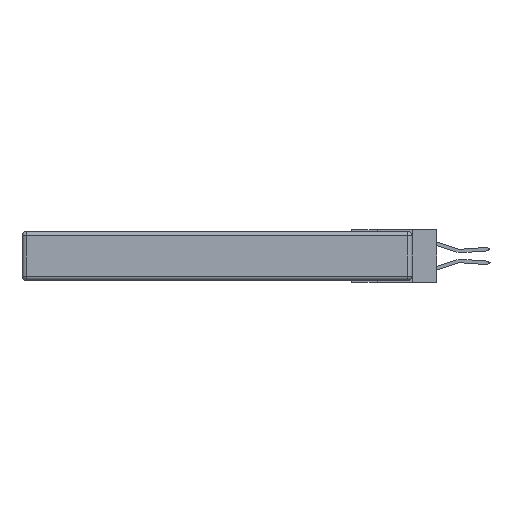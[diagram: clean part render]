
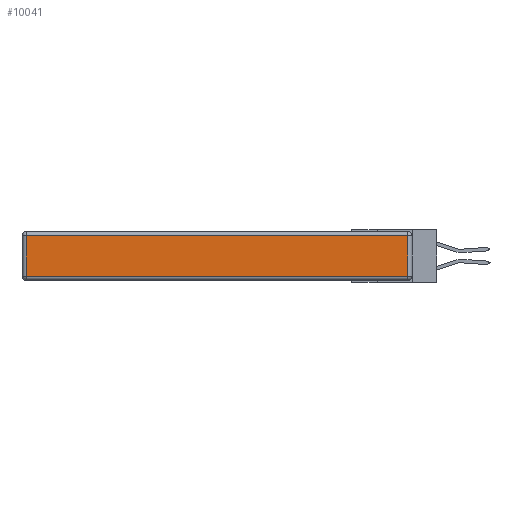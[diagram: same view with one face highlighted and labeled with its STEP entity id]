
A CAD part, left-side view. The second image highlights one B-rep face of the part: STEP entity #10041.
In plain terms, the highlighted planar face has unit normal (-1, 0, 0).
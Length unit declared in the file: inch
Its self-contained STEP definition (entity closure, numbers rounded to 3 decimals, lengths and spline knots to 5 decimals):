
#207 = CARTESIAN_POINT ( 'NONE',  ( 0., 0., -0.343 ) ) ;
#346 = LINE ( 'NONE', #9034, #8412 ) ;
#557 = ORIENTED_EDGE ( 'NONE', *, *, #4192, .T. ) ;
#729 = CARTESIAN_POINT ( 'NONE',  ( 0., 2.75, -0.03 ) ) ;
#798 = VERTEX_POINT ( 'NONE', #8414 ) ;
#1135 = FACE_OUTER_BOUND ( 'NONE', #7737, .T. ) ;
#1770 = DIRECTION ( 'NONE',  ( 0., 1., 0. ) ) ;
#1778 = EDGE_CURVE ( 'NONE', #9830, #3579, #13136, .T. ) ;
#2706 = DIRECTION ( 'NONE',  ( 0., 0., 1. ) ) ;
#3579 = VERTEX_POINT ( 'NONE', #10986 ) ;
#3909 = CARTESIAN_POINT ( 'NONE',  ( 0., 2.72, -0.343 ) ) ;
#4192 = EDGE_CURVE ( 'NONE', #798, #13851, #4459, .T. ) ;
#4459 = LINE ( 'NONE', #3909, #13299 ) ;
#5035 = EDGE_CURVE ( 'NONE', #13851, #9830, #346, .T. ) ;
#5189 = VECTOR ( 'NONE', #2706, 39.37008 ) ;
#6120 = CARTESIAN_POINT ( 'NONE',  ( 0., 0.03, -0.343 ) ) ;
#6155 = ORIENTED_EDGE ( 'NONE', *, *, #5035, .T. ) ;
#6741 = AXIS2_PLACEMENT_3D ( 'NONE', #207, #6930, #10423 ) ;
#6930 = DIRECTION ( 'NONE',  ( -1., 0., 0. ) ) ;
#7737 = EDGE_LOOP ( 'NONE', ( #6155, #11279, #12709, #557 ) ) ;
#8412 = VECTOR ( 'NONE', #10199, 39.37008 ) ;
#8414 = CARTESIAN_POINT ( 'NONE',  ( 0., 2.72, -0.03 ) ) ;
#9034 = CARTESIAN_POINT ( 'NONE',  ( 0., 0., -0.313 ) ) ;
#9527 = CARTESIAN_POINT ( 'NONE',  ( 0., 0.03, -0.313 ) ) ;
#9830 = VERTEX_POINT ( 'NONE', #9527 ) ;
#10041 = ADVANCED_FACE ( 'NONE', ( #1135 ), #10382, .T. ) ;
#10199 = DIRECTION ( 'NONE',  ( 0., -1., 0. ) ) ;
#10382 = PLANE ( 'NONE',  #6741 ) ;
#10423 = DIRECTION ( 'NONE',  ( 0., 0., 1. ) ) ;
#10986 = CARTESIAN_POINT ( 'NONE',  ( 0., 0.03, -0.03 ) ) ;
#11142 = EDGE_CURVE ( 'NONE', #3579, #798, #11915, .T. ) ;
#11279 = ORIENTED_EDGE ( 'NONE', *, *, #1778, .T. ) ;
#11627 = CARTESIAN_POINT ( 'NONE',  ( 0., 2.72, -0.313 ) ) ;
#11915 = LINE ( 'NONE', #729, #12652 ) ;
#12146 = DIRECTION ( 'NONE',  ( 0., 0., -1. ) ) ;
#12652 = VECTOR ( 'NONE', #1770, 39.37008 ) ;
#12709 = ORIENTED_EDGE ( 'NONE', *, *, #11142, .T. ) ;
#13136 = LINE ( 'NONE', #6120, #5189 ) ;
#13299 = VECTOR ( 'NONE', #12146, 39.37008 ) ;
#13851 = VERTEX_POINT ( 'NONE', #11627 ) ;
